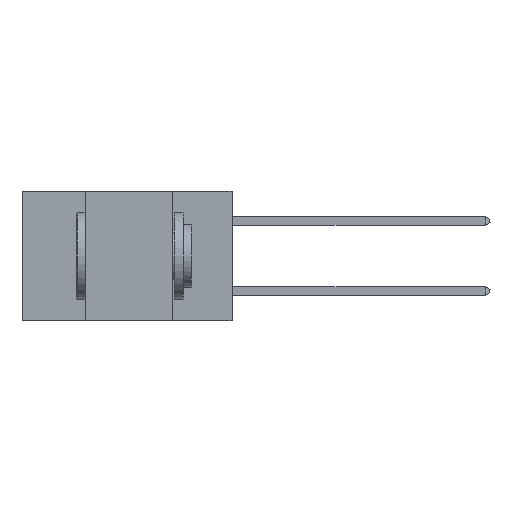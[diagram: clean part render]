
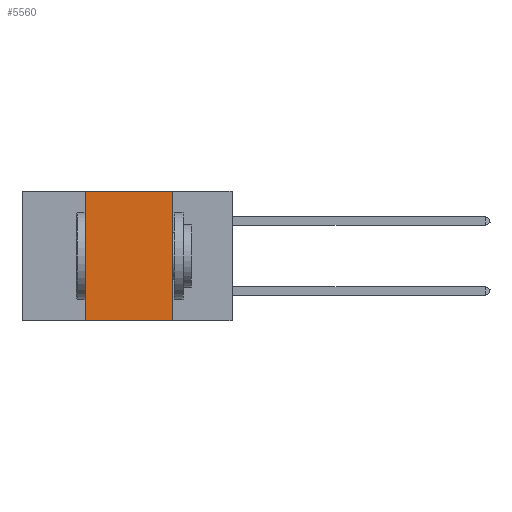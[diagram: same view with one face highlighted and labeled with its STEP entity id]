
A CAD part, left-side view. The second image highlights one B-rep face of the part: STEP entity #5560.
In plain terms, the highlighted planar face has unit normal (-1, 0, 0).
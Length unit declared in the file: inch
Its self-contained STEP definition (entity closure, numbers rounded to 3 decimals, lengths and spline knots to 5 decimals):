
#1125 = VECTOR ( 'NONE', #13287, 39.37008 ) ;
#1309 = ORIENTED_EDGE ( 'NONE', *, *, #28584, .F. ) ;
#1376 = CARTESIAN_POINT ( 'NONE',  ( 0., 0.42, -0.37 ) ) ;
#1565 = VECTOR ( 'NONE', #23544, 39.37008 ) ;
#3727 = EDGE_CURVE ( 'NONE', #21450, #33178, #23115, .T. ) ;
#4694 = VERTEX_POINT ( 'NONE', #14601 ) ;
#4731 = PLANE ( 'NONE',  #10683 ) ;
#5560 = ADVANCED_FACE ( 'NONE', ( #30168 ), #4731, .F. ) ;
#7126 = CARTESIAN_POINT ( 'NONE',  ( 0., 0.17, 0. ) ) ;
#7509 = DIRECTION ( 'NONE',  ( 1., 0., 0. ) ) ;
#10683 = AXIS2_PLACEMENT_3D ( 'NONE', #18548, #7509, #26686 ) ;
#11016 = EDGE_LOOP ( 'NONE', ( #13519, #1309, #16137, #18731 ) ) ;
#13287 = DIRECTION ( 'NONE',  ( 0., -1., 0. ) ) ;
#13519 = ORIENTED_EDGE ( 'NONE', *, *, #18633, .F. ) ;
#14468 = DIRECTION ( 'NONE',  ( 0., 0., -1. ) ) ;
#14601 = CARTESIAN_POINT ( 'NONE',  ( 0., 0.17, -0.37 ) ) ;
#16137 = ORIENTED_EDGE ( 'NONE', *, *, #3727, .F. ) ;
#17138 = CARTESIAN_POINT ( 'NONE',  ( 0., 0.17, 0. ) ) ;
#18092 = CARTESIAN_POINT ( 'NONE',  ( 0., 0.6, 0. ) ) ;
#18422 = CARTESIAN_POINT ( 'NONE',  ( 0., 0.42, 0. ) ) ;
#18548 = CARTESIAN_POINT ( 'NONE',  ( 0., 0.6, 0. ) ) ;
#18633 = EDGE_CURVE ( 'NONE', #31433, #4694, #31359, .T. ) ;
#18731 = ORIENTED_EDGE ( 'NONE', *, *, #24739, .T. ) ;
#20236 = CARTESIAN_POINT ( 'NONE',  ( 0., 0.42, 0. ) ) ;
#21450 = VERTEX_POINT ( 'NONE', #1376 ) ;
#23115 = LINE ( 'NONE', #18422, #28607 ) ;
#23544 = DIRECTION ( 'NONE',  ( 0., -1., 0. ) ) ;
#23633 = LINE ( 'NONE', #18092, #1565 ) ;
#24179 = CARTESIAN_POINT ( 'NONE',  ( 0., 0.6, -0.37 ) ) ;
#24182 = VECTOR ( 'NONE', #14468, 39.37008 ) ;
#24739 = EDGE_CURVE ( 'NONE', #21450, #4694, #30379, .T. ) ;
#26686 = DIRECTION ( 'NONE',  ( 0., 0., -1. ) ) ;
#28584 = EDGE_CURVE ( 'NONE', #33178, #31433, #23633, .T. ) ;
#28607 = VECTOR ( 'NONE', #29294, 39.37008 ) ;
#29294 = DIRECTION ( 'NONE',  ( 0., 0., 1. ) ) ;
#30168 = FACE_OUTER_BOUND ( 'NONE', #11016, .T. ) ;
#30379 = LINE ( 'NONE', #24179, #1125 ) ;
#31359 = LINE ( 'NONE', #17138, #24182 ) ;
#31433 = VERTEX_POINT ( 'NONE', #7126 ) ;
#33178 = VERTEX_POINT ( 'NONE', #20236 ) ;
